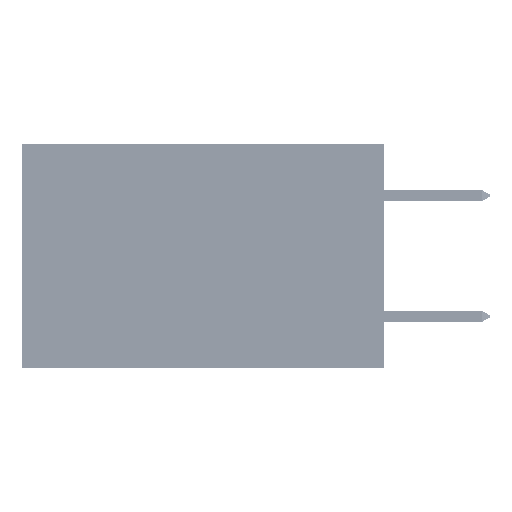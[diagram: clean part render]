
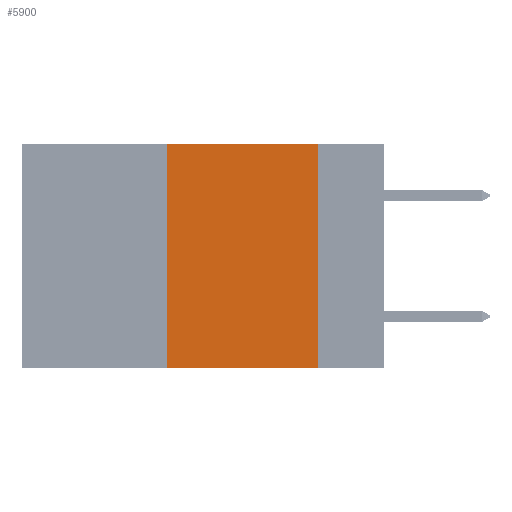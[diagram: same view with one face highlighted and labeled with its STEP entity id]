
A CAD part, left-side view. The second image highlights one B-rep face of the part: STEP entity #5900.
In plain terms, the highlighted planar face has unit normal (-1, 0, 0).
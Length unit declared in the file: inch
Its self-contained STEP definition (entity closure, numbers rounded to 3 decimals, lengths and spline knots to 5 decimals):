
#1209 = LINE ( 'NONE', #33944, #12046 ) ;
#1475 = LINE ( 'NONE', #28123, #51683 ) ;
#3985 = AXIS2_PLACEMENT_3D ( 'NONE', #11078, #27091, #19079 ) ;
#4201 = CARTESIAN_POINT ( 'NONE',  ( 4.5375, 0.05, -0.2975 ) ) ;
#5635 = VERTEX_POINT ( 'NONE', #4201 ) ;
#5900 = ADVANCED_FACE ( 'NONE', ( #51761 ), #14473, .F. ) ;
#6799 = CARTESIAN_POINT ( 'NONE',  ( 4.5375, 0.05, -0.2725 ) ) ;
#7909 = EDGE_CURVE ( 'NONE', #26666, #19231, #40913, .T. ) ;
#9804 = EDGE_LOOP ( 'NONE', ( #14436, #13073, #16697, #37729 ) ) ;
#11078 = CARTESIAN_POINT ( 'NONE',  ( 0., 0.6, 0. ) ) ;
#12046 = VECTOR ( 'NONE', #45846, 39.37008 ) ;
#13073 = ORIENTED_EDGE ( 'NONE', *, *, #27032, .F. ) ;
#13720 = DIRECTION ( 'NONE',  ( 0., -1., 0. ) ) ;
#14436 = ORIENTED_EDGE ( 'NONE', *, *, #33898, .F. ) ;
#14473 = PLANE ( 'NONE',  #3985 ) ;
#15677 = DIRECTION ( 'NONE',  ( 0., 0., 1. ) ) ;
#16165 = CARTESIAN_POINT ( 'NONE',  ( 0., 0.36, 0. ) ) ;
#16417 = VECTOR ( 'NONE', #13720, 39.37008 ) ;
#16697 = ORIENTED_EDGE ( 'NONE', *, *, #7909, .F. ) ;
#19079 = DIRECTION ( 'NONE',  ( 0., 0., -1. ) ) ;
#19231 = VERTEX_POINT ( 'NONE', #41000 ) ;
#20448 = DIRECTION ( 'NONE',  ( 0., 0., 1. ) ) ;
#26666 = VERTEX_POINT ( 'NONE', #36301 ) ;
#27032 = EDGE_CURVE ( 'NONE', #19231, #30442, #39322, .T. ) ;
#27091 = DIRECTION ( 'NONE',  ( 1., 0., 0. ) ) ;
#28123 = CARTESIAN_POINT ( 'NONE',  ( 4.5375, 0.05, -0.37 ) ) ;
#30402 = CARTESIAN_POINT ( 'NONE',  ( 0., 0.11, -0.37 ) ) ;
#30442 = VERTEX_POINT ( 'NONE', #42794 ) ;
#33898 = EDGE_CURVE ( 'NONE', #30442, #49014, #1209, .T. ) ;
#33944 = CARTESIAN_POINT ( 'NONE',  ( 0., 0.11, 0. ) ) ;
#36301 = CARTESIAN_POINT ( 'NONE',  ( 0., 0.36, -0.37 ) ) ;
#36393 = VERTEX_POINT ( 'NONE', #6799 ) ;
#37729 = EDGE_CURVE ( 'NONE', #5635, #36393, #1475, .T. ) ;
#39007 = VECTOR ( 'NONE', #20448, 39.37008 ) ;
#39322 = LINE ( 'NONE', #42110, #16417 ) ;
#40913 = LINE ( 'NONE', #16165, #39007 ) ;
#41000 = CARTESIAN_POINT ( 'NONE',  ( 0., 0.36, 0. ) ) ;
#42110 = CARTESIAN_POINT ( 'NONE',  ( 0., 0.6, 0. ) ) ;
#42794 = CARTESIAN_POINT ( 'NONE',  ( 0., 0.11, 0. ) ) ;
#45846 = DIRECTION ( 'NONE',  ( 0., 0., -1. ) ) ;
#49014 = VERTEX_POINT ( 'NONE', #30402 ) ;
#51683 = VECTOR ( 'NONE', #15677, 39.37008 ) ;
#51761 = FACE_OUTER_BOUND ( 'NONE', #9804, .T. ) ;
